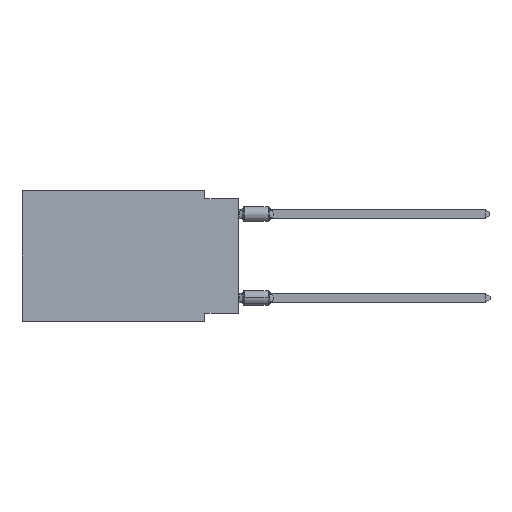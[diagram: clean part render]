
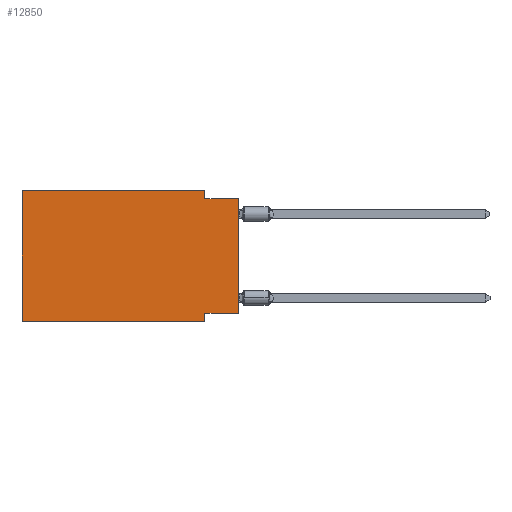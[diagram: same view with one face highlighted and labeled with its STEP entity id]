
A CAD part, left-side view. The second image highlights one B-rep face of the part: STEP entity #12850.
In plain terms, the highlighted planar face has unit normal (-1, 0, 0).
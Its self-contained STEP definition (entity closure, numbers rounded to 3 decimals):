
#97 = LINE ( 'NONE', #16736, #1606 ) ;
#953 = CARTESIAN_POINT ( 'NONE',  ( 0., 16.383, -9.906 ) ) ;
#1097 = EDGE_LOOP ( 'NONE', ( #17561, #26934, #15005, #6057, #23997, #26868, #7192, #20532 ) ) ;
#1570 = DIRECTION ( 'NONE',  ( 0., 0., 1. ) ) ;
#1606 = VECTOR ( 'NONE', #25070, 1000. ) ;
#1728 = CARTESIAN_POINT ( 'NONE',  ( 0., 2.54, -0.635 ) ) ;
#2078 = CARTESIAN_POINT ( 'NONE',  ( 0., 0., -0.635 ) ) ;
#2128 = EDGE_CURVE ( 'NONE', #20054, #10761, #26948, .T. ) ;
#2180 = CARTESIAN_POINT ( 'NONE',  ( 0., 16.383, -9.906 ) ) ;
#2426 = VECTOR ( 'NONE', #6819, 1000. ) ;
#2604 = VERTEX_POINT ( 'NONE', #2078 ) ;
#3031 = CARTESIAN_POINT ( 'NONE',  ( 0., 2.54, -9.906 ) ) ;
#3247 = VERTEX_POINT ( 'NONE', #953 ) ;
#3602 = AXIS2_PLACEMENT_3D ( 'NONE', #3615, #9353, #7573 ) ;
#3615 = CARTESIAN_POINT ( 'NONE',  ( 0., 16.383, 0. ) ) ;
#3744 = CARTESIAN_POINT ( 'NONE',  ( 0., 0., -9.271 ) ) ;
#4360 = EDGE_CURVE ( 'NONE', #3247, #6847, #11917, .T. ) ;
#4416 = EDGE_CURVE ( 'NONE', #18339, #2604, #22984, .T. ) ;
#5666 = FACE_OUTER_BOUND ( 'NONE', #1097, .T. ) ;
#6057 = ORIENTED_EDGE ( 'NONE', *, *, #13442, .F. ) ;
#6136 = CARTESIAN_POINT ( 'NONE',  ( 0., 16.383, 0. ) ) ;
#6331 = CARTESIAN_POINT ( 'NONE',  ( 0., 0., -0.635 ) ) ;
#6570 = CARTESIAN_POINT ( 'NONE',  ( 0., 2.54, 0. ) ) ;
#6705 = LINE ( 'NONE', #6570, #26358 ) ;
#6819 = DIRECTION ( 'NONE',  ( 0., -1., 0. ) ) ;
#6847 = VERTEX_POINT ( 'NONE', #20168 ) ;
#7192 = ORIENTED_EDGE ( 'NONE', *, *, #15777, .F. ) ;
#7543 = CARTESIAN_POINT ( 'NONE',  ( 0., 2.54, -9.906 ) ) ;
#7573 = DIRECTION ( 'NONE',  ( 0., 0., -1. ) ) ;
#9353 = DIRECTION ( 'NONE',  ( 1., 0., 0. ) ) ;
#10298 = EDGE_CURVE ( 'NONE', #19273, #18339, #6705, .T. ) ;
#10761 = VERTEX_POINT ( 'NONE', #21087 ) ;
#11917 = LINE ( 'NONE', #20253, #20311 ) ;
#12850 = ADVANCED_FACE ( 'NONE', ( #5666 ), #22308, .F. ) ;
#13442 = EDGE_CURVE ( 'NONE', #6847, #19273, #25369, .T. ) ;
#14309 = VECTOR ( 'NONE', #24618, 1000. ) ;
#14851 = DIRECTION ( 'NONE',  ( 0., -1., 0. ) ) ;
#15005 = ORIENTED_EDGE ( 'NONE', *, *, #10298, .F. ) ;
#15777 = EDGE_CURVE ( 'NONE', #10761, #20596, #18572, .T. ) ;
#16289 = CARTESIAN_POINT ( 'NONE',  ( 0., 0., -9.271 ) ) ;
#16736 = CARTESIAN_POINT ( 'NONE',  ( 0., 0., 0. ) ) ;
#16910 = LINE ( 'NONE', #2180, #2426 ) ;
#16935 = EDGE_CURVE ( 'NONE', #20054, #2604, #97, .T. ) ;
#17259 = VECTOR ( 'NONE', #19418, 1000. ) ;
#17561 = ORIENTED_EDGE ( 'NONE', *, *, #16935, .T. ) ;
#17567 = VECTOR ( 'NONE', #14851, 1000. ) ;
#18339 = VERTEX_POINT ( 'NONE', #1728 ) ;
#18572 = LINE ( 'NONE', #7543, #19778 ) ;
#18839 = DIRECTION ( 'NONE',  ( 0., 0., -1. ) ) ;
#19273 = VERTEX_POINT ( 'NONE', #26891 ) ;
#19418 = DIRECTION ( 'NONE',  ( 0., -1., 0. ) ) ;
#19778 = VECTOR ( 'NONE', #25756, 1000. ) ;
#20054 = VERTEX_POINT ( 'NONE', #3744 ) ;
#20168 = CARTESIAN_POINT ( 'NONE',  ( 0., 16.383, 0. ) ) ;
#20253 = CARTESIAN_POINT ( 'NONE',  ( 0., 16.383, 0. ) ) ;
#20311 = VECTOR ( 'NONE', #1570, 1000. ) ;
#20532 = ORIENTED_EDGE ( 'NONE', *, *, #2128, .F. ) ;
#20596 = VERTEX_POINT ( 'NONE', #3031 ) ;
#20897 = EDGE_CURVE ( 'NONE', #3247, #20596, #16910, .T. ) ;
#21087 = CARTESIAN_POINT ( 'NONE',  ( 0., 2.54, -9.271 ) ) ;
#22308 = PLANE ( 'NONE',  #3602 ) ;
#22984 = LINE ( 'NONE', #6331, #17259 ) ;
#23997 = ORIENTED_EDGE ( 'NONE', *, *, #4360, .F. ) ;
#24618 = DIRECTION ( 'NONE',  ( 0., 1., 0. ) ) ;
#25070 = DIRECTION ( 'NONE',  ( 0., 0., 1. ) ) ;
#25369 = LINE ( 'NONE', #6136, #17567 ) ;
#25756 = DIRECTION ( 'NONE',  ( 0., 0., -1. ) ) ;
#26358 = VECTOR ( 'NONE', #18839, 1000. ) ;
#26868 = ORIENTED_EDGE ( 'NONE', *, *, #20897, .T. ) ;
#26891 = CARTESIAN_POINT ( 'NONE',  ( 0., 2.54, 0. ) ) ;
#26934 = ORIENTED_EDGE ( 'NONE', *, *, #4416, .F. ) ;
#26948 = LINE ( 'NONE', #16289, #14309 ) ;
